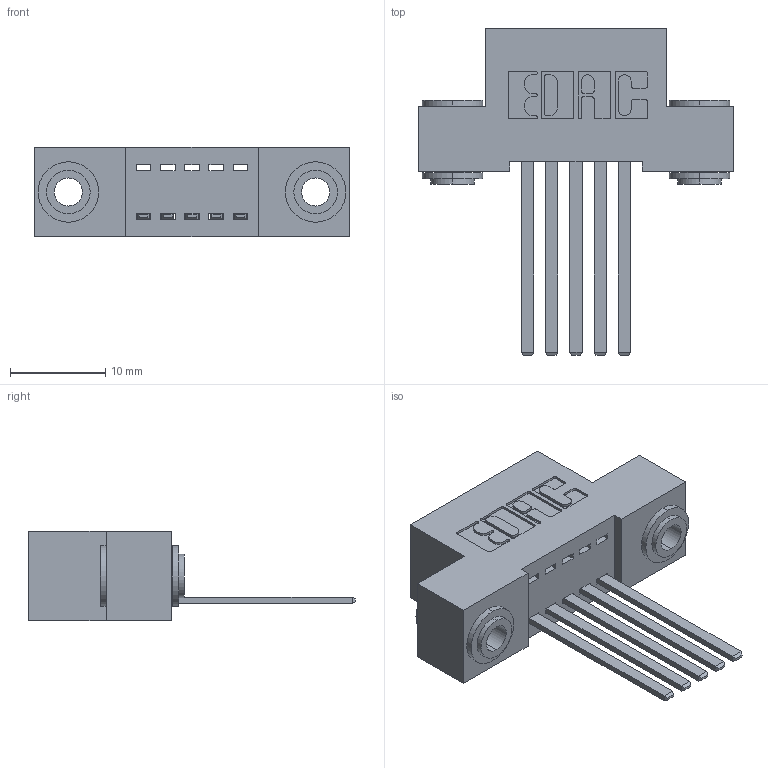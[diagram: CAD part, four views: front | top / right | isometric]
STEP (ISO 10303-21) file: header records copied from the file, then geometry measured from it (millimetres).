
FILE_DESCRIPTION (( 'STEP AP203' ), '1' );
FILE_NAME ('342-005-544-103.STEP', '2019-10-01T12:18:53', ( '' ), ( '' ), 'SwSTEP 2.0', 'SolidWorks 2016', '' );
FILE_SCHEMA (( 'CONFIG_CONTROL_DESIGN' ));
Length unit declared in the file: inch
Products named in the file (4): 342 Part_.156 TH; 345-292-001_345-293-144; 342-250-002_345-250-002-102; 342-005-544-103
Assembly tree (8 placements, depth 2):
  342-005-544-103
    342 Part_.156 TH
    345-292-001_345-293-144  x5
    342-250-002_345-250-002-102  x2
Bounding box: 33.02 x 34.3 x 9.4 mm (x, y, z)
Volume: 2839.6 mm3; surface area: 3870 mm2
Topology: 8 solids, 8 shells, 408 faces, 1165 edges, 766 vertices
Faces by surface type: plane 266, cylinder 134, cone 8
Entity records: 8176 total; most frequent: CARTESIAN_POINT 1392, ORIENTED_EDGE 1326, DIRECTION 1279, EDGE_CURVE 663, LINE 515, VECTOR 515, VERTEX_POINT 438, AXIS2_PLACEMENT_3D 382
